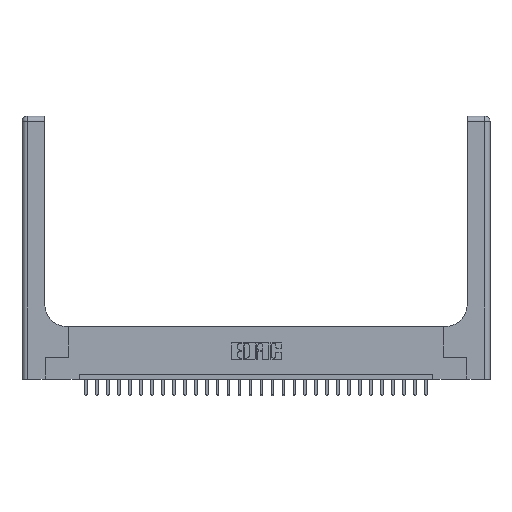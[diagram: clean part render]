
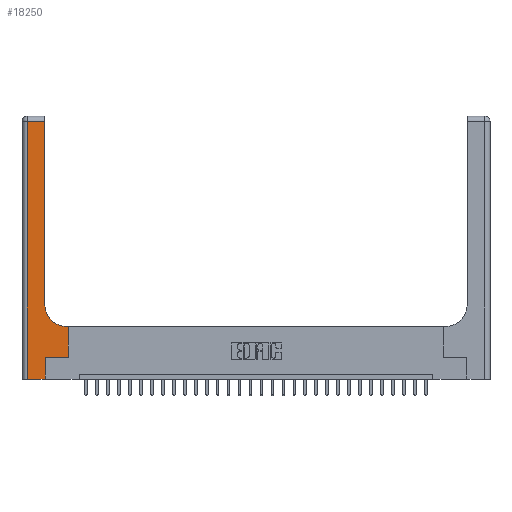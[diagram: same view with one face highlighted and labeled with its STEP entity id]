
A CAD part, top view. The second image highlights one B-rep face of the part: STEP entity #18250.
In plain terms, the highlighted planar face has unit normal (0, 0, 1).
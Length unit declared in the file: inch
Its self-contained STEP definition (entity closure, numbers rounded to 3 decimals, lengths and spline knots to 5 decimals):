
#822 = CARTESIAN_POINT ( 'NONE',  ( 0.265, 0.25, 0.37 ) ) ;
#1434 = CARTESIAN_POINT ( 'NONE',  ( 0.265, 0., 0.37 ) ) ;
#1782 = LINE ( 'NONE', #10945, #9144 ) ;
#1840 = VECTOR ( 'NONE', #3055, 39.37008 ) ;
#2832 = ORIENTED_EDGE ( 'NONE', *, *, #3432, .T. ) ;
#3055 = DIRECTION ( 'NONE',  ( 1., 0., 0. ) ) ;
#3271 = EDGE_CURVE ( 'NONE', #23725, #18550, #16636, .T. ) ;
#3308 = EDGE_CURVE ( 'NONE', #20820, #15900, #14376, .T. ) ;
#3370 = EDGE_CURVE ( 'NONE', #12216, #23725, #9546, .T. ) ;
#3432 = EDGE_CURVE ( 'NONE', #9132, #12788, #19232, .T. ) ;
#3678 = CARTESIAN_POINT ( 'NONE',  ( 0.265, 0., 0.37 ) ) ;
#4182 = EDGE_CURVE ( 'NONE', #15900, #16028, #16251, .T. ) ;
#5539 = DIRECTION ( 'NONE',  ( 0., 1., 0. ) ) ;
#5604 = VECTOR ( 'NONE', #14318, 39.37008 ) ;
#5852 = AXIS2_PLACEMENT_3D ( 'NONE', #25943, #9610, #15753 ) ;
#6270 = DIRECTION ( 'NONE',  ( 0., 1., 0. ) ) ;
#6335 = CARTESIAN_POINT ( 'NONE',  ( 0.528, 0.6, 0.37 ) ) ;
#7485 = CARTESIAN_POINT ( 'NONE',  ( 0.528, 0.25, 0.37 ) ) ;
#7630 = ORIENTED_EDGE ( 'NONE', *, *, #3308, .T. ) ;
#7818 = CARTESIAN_POINT ( 'NONE',  ( 0., 2.94, 0.37 ) ) ;
#7968 = ORIENTED_EDGE ( 'NONE', *, *, #3271, .T. ) ;
#8182 = CARTESIAN_POINT ( 'NONE',  ( 0.26, 0.85, 0.37 ) ) ;
#9074 = ORIENTED_EDGE ( 'NONE', *, *, #4182, .T. ) ;
#9132 = VERTEX_POINT ( 'NONE', #9962 ) ;
#9144 = VECTOR ( 'NONE', #25208, 39.37008 ) ;
#9342 = CARTESIAN_POINT ( 'NONE',  ( 0.528, 0.25, 0.37 ) ) ;
#9446 = CARTESIAN_POINT ( 'NONE',  ( 0.06, 3., 0.37 ) ) ;
#9546 = LINE ( 'NONE', #1434, #20172 ) ;
#9610 = DIRECTION ( 'NONE',  ( 0., 0., -1. ) ) ;
#9962 = CARTESIAN_POINT ( 'NONE',  ( 0.06, 2.94, 0.37 ) ) ;
#10576 = CARTESIAN_POINT ( 'NONE',  ( 0.06, 0., 0.37 ) ) ;
#10945 = CARTESIAN_POINT ( 'NONE',  ( 0., 0., 0.37 ) ) ;
#11692 = LINE ( 'NONE', #7818, #5604 ) ;
#11848 = CARTESIAN_POINT ( 'NONE',  ( 0.51, 0.6, 0.37 ) ) ;
#12016 = EDGE_CURVE ( 'NONE', #12788, #12216, #1782, .T. ) ;
#12216 = VERTEX_POINT ( 'NONE', #3678 ) ;
#12788 = VERTEX_POINT ( 'NONE', #10576 ) ;
#14055 = VECTOR ( 'NONE', #24080, 39.37008 ) ;
#14310 = FACE_OUTER_BOUND ( 'NONE', #18004, .T. ) ;
#14318 = DIRECTION ( 'NONE',  ( -1., 0., 0. ) ) ;
#14376 = CIRCLE ( 'NONE', #17330, 0.25 ) ;
#14622 = ORIENTED_EDGE ( 'NONE', *, *, #19345, .T. ) ;
#15081 = DIRECTION ( 'NONE',  ( 0., 0., -1. ) ) ;
#15753 = DIRECTION ( 'NONE',  ( -1., 0., 0. ) ) ;
#15900 = VERTEX_POINT ( 'NONE', #8182 ) ;
#16028 = VERTEX_POINT ( 'NONE', #24613 ) ;
#16251 = LINE ( 'NONE', #18616, #23946 ) ;
#16303 = LINE ( 'NONE', #22902, #26527 ) ;
#16636 = LINE ( 'NONE', #822, #1840 ) ;
#16821 = ORIENTED_EDGE ( 'NONE', *, *, #3370, .T. ) ;
#16958 = EDGE_CURVE ( 'NONE', #20919, #20820, #16303, .T. ) ;
#17034 = DIRECTION ( 'NONE',  ( -1., 0., 0. ) ) ;
#17318 = CARTESIAN_POINT ( 'NONE',  ( 0.51, 0.85, 0.37 ) ) ;
#17330 = AXIS2_PLACEMENT_3D ( 'NONE', #17318, #15081, #19737 ) ;
#18004 = EDGE_LOOP ( 'NONE', ( #9074, #14622, #2832, #26284, #16821, #7968, #19708, #24689, #7630 ) ) ;
#18250 = ADVANCED_FACE ( 'NONE', ( #14310 ), #26021, .F. ) ;
#18550 = VERTEX_POINT ( 'NONE', #9342 ) ;
#18616 = CARTESIAN_POINT ( 'NONE',  ( 0.26, 3., 0.37 ) ) ;
#19232 = LINE ( 'NONE', #9446, #14055 ) ;
#19345 = EDGE_CURVE ( 'NONE', #16028, #9132, #11692, .T. ) ;
#19708 = ORIENTED_EDGE ( 'NONE', *, *, #26427, .T. ) ;
#19737 = DIRECTION ( 'NONE',  ( 1., 0., 0. ) ) ;
#20172 = VECTOR ( 'NONE', #5539, 39.37008 ) ;
#20820 = VERTEX_POINT ( 'NONE', #11848 ) ;
#20919 = VERTEX_POINT ( 'NONE', #6335 ) ;
#22902 = CARTESIAN_POINT ( 'NONE',  ( 0.26, 0.6, 0.37 ) ) ;
#23645 = LINE ( 'NONE', #7485, #26498 ) ;
#23725 = VERTEX_POINT ( 'NONE', #25153 ) ;
#23936 = DIRECTION ( 'NONE',  ( 0., 1., 0. ) ) ;
#23946 = VECTOR ( 'NONE', #6270, 39.37008 ) ;
#24080 = DIRECTION ( 'NONE',  ( 0., -1., 0. ) ) ;
#24613 = CARTESIAN_POINT ( 'NONE',  ( 0.26, 2.94, 0.37 ) ) ;
#24689 = ORIENTED_EDGE ( 'NONE', *, *, #16958, .T. ) ;
#25153 = CARTESIAN_POINT ( 'NONE',  ( 0.265, 0.25, 0.37 ) ) ;
#25208 = DIRECTION ( 'NONE',  ( 1., 0., 0. ) ) ;
#25943 = CARTESIAN_POINT ( 'NONE',  ( 0., 3., 0.37 ) ) ;
#26021 = PLANE ( 'NONE',  #5852 ) ;
#26284 = ORIENTED_EDGE ( 'NONE', *, *, #12016, .T. ) ;
#26427 = EDGE_CURVE ( 'NONE', #18550, #20919, #23645, .T. ) ;
#26498 = VECTOR ( 'NONE', #23936, 39.37008 ) ;
#26527 = VECTOR ( 'NONE', #17034, 39.37008 ) ;
